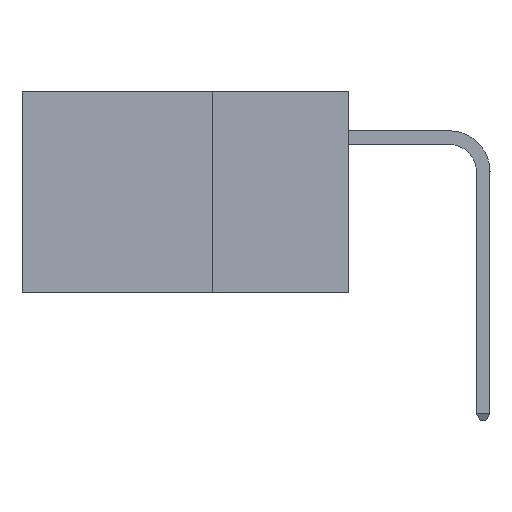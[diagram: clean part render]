
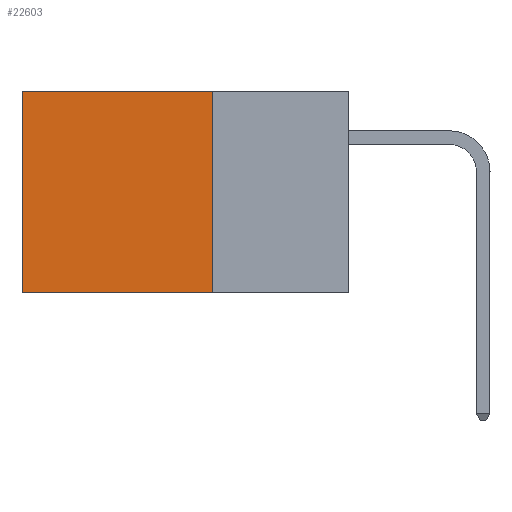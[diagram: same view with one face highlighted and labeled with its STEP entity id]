
A CAD part, left-side view. The second image highlights one B-rep face of the part: STEP entity #22603.
In plain terms, the highlighted planar face has unit normal (-1, 0, 0).
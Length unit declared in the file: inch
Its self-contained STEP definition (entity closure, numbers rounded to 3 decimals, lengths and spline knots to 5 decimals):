
#2989 = LINE ( 'NONE', #37474, #29408 ) ;
#3867 = CARTESIAN_POINT ( 'NONE',  ( 0.2875, 0.25, -0.37 ) ) ;
#4859 = ORIENTED_EDGE ( 'NONE', *, *, #37832, .F. ) ;
#6100 = VECTOR ( 'NONE', #43636, 39.37008 ) ;
#7704 = DIRECTION ( 'NONE',  ( 1., 0., 0. ) ) ;
#8835 = EDGE_CURVE ( 'NONE', #12192, #26218, #15740, .T. ) ;
#10247 = ORIENTED_EDGE ( 'NONE', *, *, #38042, .F. ) ;
#10699 = ORIENTED_EDGE ( 'NONE', *, *, #8835, .T. ) ;
#11199 = PLANE ( 'NONE',  #41140 ) ;
#12192 = VERTEX_POINT ( 'NONE', #42022 ) ;
#12897 = VECTOR ( 'NONE', #33270, 39.37008 ) ;
#14209 = ORIENTED_EDGE ( 'NONE', *, *, #25511, .T. ) ;
#15740 = LINE ( 'NONE', #36458, #6100 ) ;
#22603 = ADVANCED_FACE ( 'NONE', ( #36348 ), #11199, .F. ) ;
#24065 = LINE ( 'NONE', #30605, #43071 ) ;
#24110 = EDGE_LOOP ( 'NONE', ( #10699, #4859, #10247, #14209 ) ) ;
#25511 = EDGE_CURVE ( 'NONE', #35615, #12192, #2989, .T. ) ;
#26218 = VERTEX_POINT ( 'NONE', #27081 ) ;
#27081 = CARTESIAN_POINT ( 'NONE',  ( 0.2875, 0.6, -0.37 ) ) ;
#29173 = CARTESIAN_POINT ( 'NONE',  ( 0.2875, 0.25, 0. ) ) ;
#29408 = VECTOR ( 'NONE', #30427, 39.37008 ) ;
#30427 = DIRECTION ( 'NONE',  ( 0., 1., 0. ) ) ;
#30605 = CARTESIAN_POINT ( 'NONE',  ( 0.2875, 0.25, 0. ) ) ;
#32770 = DIRECTION ( 'NONE',  ( 0., 0., -1. ) ) ;
#33263 = VERTEX_POINT ( 'NONE', #3867 ) ;
#33270 = DIRECTION ( 'NONE',  ( 0., 1., 0. ) ) ;
#35615 = VERTEX_POINT ( 'NONE', #42213 ) ;
#36348 = FACE_OUTER_BOUND ( 'NONE', #24110, .T. ) ;
#36458 = CARTESIAN_POINT ( 'NONE',  ( 0.2875, 0.6, 0. ) ) ;
#37474 = CARTESIAN_POINT ( 'NONE',  ( 0.2875, 0.25, 0. ) ) ;
#37832 = EDGE_CURVE ( 'NONE', #33263, #26218, #42546, .T. ) ;
#38042 = EDGE_CURVE ( 'NONE', #35615, #33263, #24065, .T. ) ;
#40297 = CARTESIAN_POINT ( 'NONE',  ( 0.2875, 0.25, -0.37 ) ) ;
#41140 = AXIS2_PLACEMENT_3D ( 'NONE', #29173, #7704, #32770 ) ;
#41387 = DIRECTION ( 'NONE',  ( 0., 0., -1. ) ) ;
#42022 = CARTESIAN_POINT ( 'NONE',  ( 0.2875, 0.6, 0. ) ) ;
#42213 = CARTESIAN_POINT ( 'NONE',  ( 0.2875, 0.25, 0. ) ) ;
#42546 = LINE ( 'NONE', #40297, #12897 ) ;
#43071 = VECTOR ( 'NONE', #41387, 39.37008 ) ;
#43636 = DIRECTION ( 'NONE',  ( 0., 0., -1. ) ) ;
